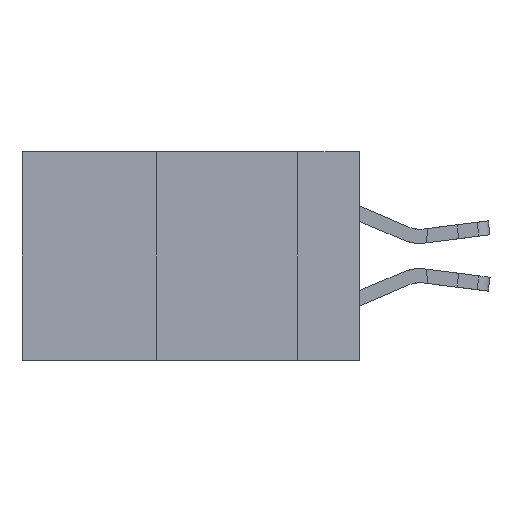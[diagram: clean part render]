
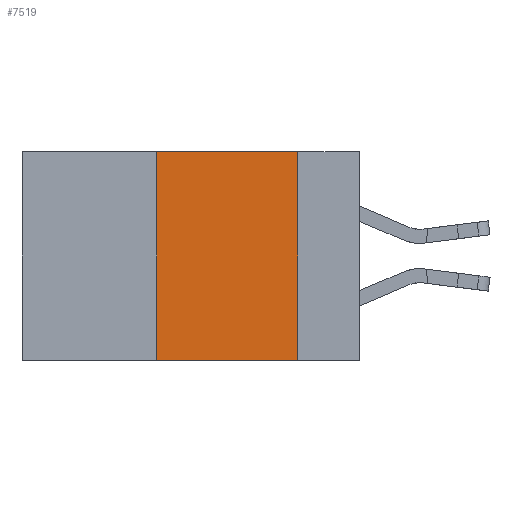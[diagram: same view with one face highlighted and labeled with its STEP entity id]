
A CAD part, left-side view. The second image highlights one B-rep face of the part: STEP entity #7519.
In plain terms, the highlighted planar face has unit normal (-1, 0, 0).
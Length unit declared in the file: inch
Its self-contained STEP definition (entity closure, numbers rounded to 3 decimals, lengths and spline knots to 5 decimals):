
#2068 = EDGE_CURVE ( 'NONE', #18031, #20664, #11838, .T. ) ;
#3064 = VERTEX_POINT ( 'NONE', #18746 ) ;
#4178 = LINE ( 'NONE', #19747, #10695 ) ;
#4351 = CARTESIAN_POINT ( 'NONE',  ( 0., 0.36, 0. ) ) ;
#4413 = DIRECTION ( 'NONE',  ( 0., -1., 0. ) ) ;
#5561 = CARTESIAN_POINT ( 'NONE',  ( 0., 0.11, 0. ) ) ;
#6591 = LINE ( 'NONE', #19607, #8422 ) ;
#7232 = VERTEX_POINT ( 'NONE', #20739 ) ;
#7519 = ADVANCED_FACE ( 'NONE', ( #9966 ), #7792, .F. ) ;
#7792 = PLANE ( 'NONE',  #15605 ) ;
#8059 = ORIENTED_EDGE ( 'NONE', *, *, #2068, .F. ) ;
#8422 = VECTOR ( 'NONE', #14845, 39.37008 ) ;
#9553 = DIRECTION ( 'NONE',  ( 1., 0., 0. ) ) ;
#9639 = DIRECTION ( 'NONE',  ( 0., 0., 1. ) ) ;
#9843 = VECTOR ( 'NONE', #9639, 39.37008 ) ;
#9966 = FACE_OUTER_BOUND ( 'NONE', #18011, .T. ) ;
#10695 = VECTOR ( 'NONE', #19669, 39.37008 ) ;
#11719 = ORIENTED_EDGE ( 'NONE', *, *, #17086, .T. ) ;
#11838 = LINE ( 'NONE', #20911, #15734 ) ;
#14285 = LINE ( 'NONE', #14596, #9843 ) ;
#14342 = EDGE_CURVE ( 'NONE', #7232, #18031, #14285, .T. ) ;
#14596 = CARTESIAN_POINT ( 'NONE',  ( 0., 0.36, 0. ) ) ;
#14845 = DIRECTION ( 'NONE',  ( 0., -1., 0. ) ) ;
#15605 = AXIS2_PLACEMENT_3D ( 'NONE', #21252, #9553, #21176 ) ;
#15734 = VECTOR ( 'NONE', #4413, 39.37008 ) ;
#16759 = ORIENTED_EDGE ( 'NONE', *, *, #18574, .F. ) ;
#17086 = EDGE_CURVE ( 'NONE', #7232, #3064, #6591, .T. ) ;
#18011 = EDGE_LOOP ( 'NONE', ( #16759, #8059, #19534, #11719 ) ) ;
#18031 = VERTEX_POINT ( 'NONE', #4351 ) ;
#18574 = EDGE_CURVE ( 'NONE', #20664, #3064, #4178, .T. ) ;
#18746 = CARTESIAN_POINT ( 'NONE',  ( 0., 0.11, -0.37 ) ) ;
#19534 = ORIENTED_EDGE ( 'NONE', *, *, #14342, .F. ) ;
#19607 = CARTESIAN_POINT ( 'NONE',  ( 0., 0.6, -0.37 ) ) ;
#19669 = DIRECTION ( 'NONE',  ( 0., 0., -1. ) ) ;
#19747 = CARTESIAN_POINT ( 'NONE',  ( 0., 0.11, 0. ) ) ;
#20664 = VERTEX_POINT ( 'NONE', #5561 ) ;
#20739 = CARTESIAN_POINT ( 'NONE',  ( 0., 0.36, -0.37 ) ) ;
#20911 = CARTESIAN_POINT ( 'NONE',  ( 0., 0.6, 0. ) ) ;
#21176 = DIRECTION ( 'NONE',  ( 0., 0., -1. ) ) ;
#21252 = CARTESIAN_POINT ( 'NONE',  ( 0., 0.6, 0. ) ) ;
